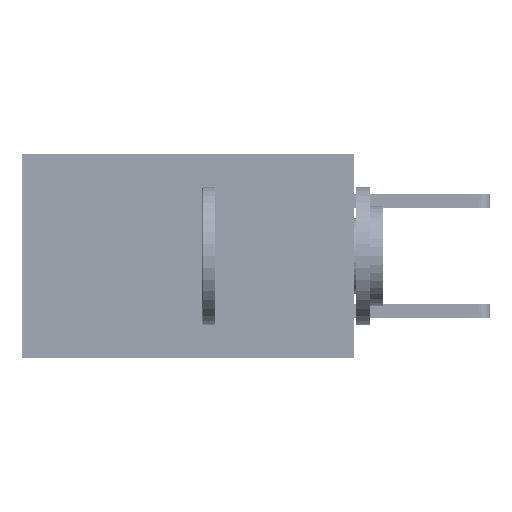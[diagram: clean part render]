
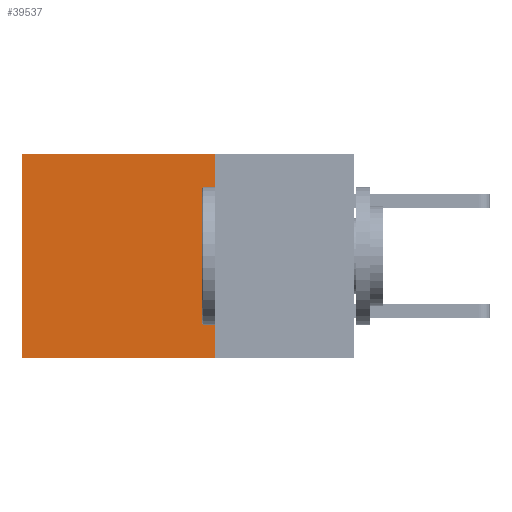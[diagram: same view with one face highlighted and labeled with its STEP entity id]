
A CAD part, left-side view. The second image highlights one B-rep face of the part: STEP entity #39537.
In plain terms, the highlighted planar face has unit normal (-1, 0, 0).
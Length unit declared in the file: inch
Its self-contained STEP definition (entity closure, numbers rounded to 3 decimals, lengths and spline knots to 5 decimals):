
#128 = EDGE_CURVE ( 'NONE', #43040, #29556, #40332, .T. ) ;
#332 = DIRECTION ( 'NONE',  ( 0., 1., 0. ) ) ;
#398 = FACE_OUTER_BOUND ( 'NONE', #40434, .T. ) ;
#1708 = EDGE_CURVE ( 'NONE', #43040, #8160, #37382, .T. ) ;
#3453 = DIRECTION ( 'NONE',  ( 0., 0., -1. ) ) ;
#3735 = VECTOR ( 'NONE', #33779, 39.37008 ) ;
#5513 = ORIENTED_EDGE ( 'NONE', *, *, #128, .F. ) ;
#7221 = CARTESIAN_POINT ( 'NONE',  ( 0.2875, 0.6, 0. ) ) ;
#8160 = VERTEX_POINT ( 'NONE', #7221 ) ;
#10742 = CARTESIAN_POINT ( 'NONE',  ( 0.2875, 0.6, -0.37 ) ) ;
#13044 = DIRECTION ( 'NONE',  ( 1., 0., 0. ) ) ;
#13660 = VECTOR ( 'NONE', #30382, 39.37008 ) ;
#16202 = PLANE ( 'NONE',  #37573 ) ;
#16253 = CARTESIAN_POINT ( 'NONE',  ( 0.2875, 0.25, 0. ) ) ;
#19065 = EDGE_CURVE ( 'NONE', #8160, #38387, #42468, .T. ) ;
#19954 = CARTESIAN_POINT ( 'NONE',  ( 0.2875, 0.25, 0. ) ) ;
#20023 = CARTESIAN_POINT ( 'NONE',  ( 0.2875, 0.25, -0.37 ) ) ;
#26754 = CARTESIAN_POINT ( 'NONE',  ( 0.2875, 0.25, -0.37 ) ) ;
#27301 = CARTESIAN_POINT ( 'NONE',  ( 0.2875, 0.25, 0. ) ) ;
#29556 = VERTEX_POINT ( 'NONE', #20023 ) ;
#29832 = LINE ( 'NONE', #26754, #13660 ) ;
#30382 = DIRECTION ( 'NONE',  ( 0., 1., 0. ) ) ;
#33779 = DIRECTION ( 'NONE',  ( 0., 0., -1. ) ) ;
#34791 = ORIENTED_EDGE ( 'NONE', *, *, #37532, .F. ) ;
#35681 = CARTESIAN_POINT ( 'NONE',  ( 0.2875, 0.25, 0. ) ) ;
#36821 = DIRECTION ( 'NONE',  ( 0., 0., -1. ) ) ;
#37382 = LINE ( 'NONE', #27301, #37892 ) ;
#37532 = EDGE_CURVE ( 'NONE', #29556, #38387, #29832, .T. ) ;
#37573 = AXIS2_PLACEMENT_3D ( 'NONE', #19954, #13044, #36821 ) ;
#37892 = VECTOR ( 'NONE', #332, 39.37008 ) ;
#38315 = ORIENTED_EDGE ( 'NONE', *, *, #19065, .T. ) ;
#38387 = VERTEX_POINT ( 'NONE', #10742 ) ;
#39251 = VECTOR ( 'NONE', #3453, 39.37008 ) ;
#39537 = ADVANCED_FACE ( 'NONE', ( #398 ), #16202, .F. ) ;
#40332 = LINE ( 'NONE', #35681, #39251 ) ;
#40434 = EDGE_LOOP ( 'NONE', ( #38315, #34791, #5513, #44352 ) ) ;
#40788 = CARTESIAN_POINT ( 'NONE',  ( 0.2875, 0.6, 0. ) ) ;
#42468 = LINE ( 'NONE', #40788, #3735 ) ;
#43040 = VERTEX_POINT ( 'NONE', #16253 ) ;
#44352 = ORIENTED_EDGE ( 'NONE', *, *, #1708, .T. ) ;
